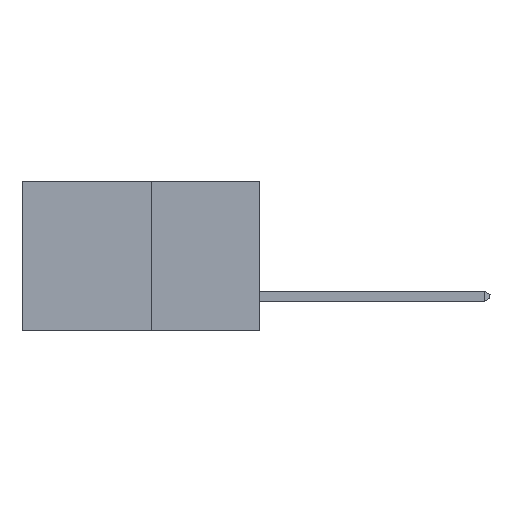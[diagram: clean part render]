
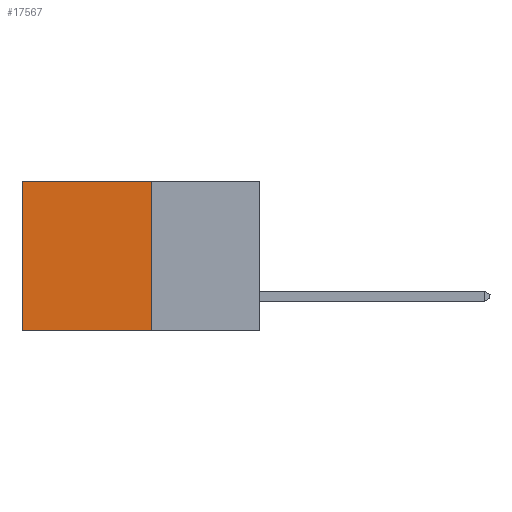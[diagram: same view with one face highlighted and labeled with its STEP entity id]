
A CAD part, left-side view. The second image highlights one B-rep face of the part: STEP entity #17567.
In plain terms, the highlighted planar face has unit normal (-1, 0, 0).
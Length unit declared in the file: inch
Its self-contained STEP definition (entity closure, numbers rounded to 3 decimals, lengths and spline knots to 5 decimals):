
#371 = CARTESIAN_POINT ( 'NONE',  ( 0.277, 0.59, 0. ) ) ;
#613 = ORIENTED_EDGE ( 'NONE', *, *, #22985, .F. ) ;
#982 = AXIS2_PLACEMENT_3D ( 'NONE', #13356, #4109, #20392 ) ;
#1443 = VECTOR ( 'NONE', #17323, 39.37008 ) ;
#1579 = VECTOR ( 'NONE', #10086, 39.37008 ) ;
#2137 = LINE ( 'NONE', #10068, #1579 ) ;
#4109 = DIRECTION ( 'NONE',  ( 1., 0., 0. ) ) ;
#4793 = CARTESIAN_POINT ( 'NONE',  ( 0.277, 0.59, -0.37 ) ) ;
#5698 = CARTESIAN_POINT ( 'NONE',  ( 0.277, 0.27, 0. ) ) ;
#8497 = EDGE_LOOP ( 'NONE', ( #13514, #21182, #613, #10067 ) ) ;
#8804 = EDGE_CURVE ( 'NONE', #21291, #21212, #9125, .T. ) ;
#9125 = LINE ( 'NONE', #29122, #25935 ) ;
#10067 = ORIENTED_EDGE ( 'NONE', *, *, #27814, .T. ) ;
#10068 = CARTESIAN_POINT ( 'NONE',  ( 0.277, 0.27, -0.37 ) ) ;
#10086 = DIRECTION ( 'NONE',  ( 0., 1., 0. ) ) ;
#10273 = EDGE_CURVE ( 'NONE', #24475, #21212, #2137, .T. ) ;
#12846 = VERTEX_POINT ( 'NONE', #28632 ) ;
#13356 = CARTESIAN_POINT ( 'NONE',  ( 0.277, 0.27, -0.37 ) ) ;
#13514 = ORIENTED_EDGE ( 'NONE', *, *, #8804, .T. ) ;
#16213 = CARTESIAN_POINT ( 'NONE',  ( 0.277, 0.27, -0.37 ) ) ;
#17323 = DIRECTION ( 'NONE',  ( 0., 1., 0. ) ) ;
#17567 = ADVANCED_FACE ( 'NONE', ( #23537 ), #17945, .F. ) ;
#17945 = PLANE ( 'NONE',  #982 ) ;
#18437 = DIRECTION ( 'NONE',  ( 0., 0., -1. ) ) ;
#18791 = LINE ( 'NONE', #16213, #24263 ) ;
#19976 = LINE ( 'NONE', #5698, #1443 ) ;
#20392 = DIRECTION ( 'NONE',  ( 0., 0., -1. ) ) ;
#21182 = ORIENTED_EDGE ( 'NONE', *, *, #10273, .F. ) ;
#21212 = VERTEX_POINT ( 'NONE', #4793 ) ;
#21291 = VERTEX_POINT ( 'NONE', #371 ) ;
#22985 = EDGE_CURVE ( 'NONE', #12846, #24475, #18791, .T. ) ;
#23537 = FACE_OUTER_BOUND ( 'NONE', #8497, .T. ) ;
#23596 = CARTESIAN_POINT ( 'NONE',  ( 0.277, 0.27, -0.37 ) ) ;
#24263 = VECTOR ( 'NONE', #18437, 39.37008 ) ;
#24475 = VERTEX_POINT ( 'NONE', #23596 ) ;
#25935 = VECTOR ( 'NONE', #29084, 39.37008 ) ;
#27814 = EDGE_CURVE ( 'NONE', #12846, #21291, #19976, .T. ) ;
#28632 = CARTESIAN_POINT ( 'NONE',  ( 0.277, 0.27, 0. ) ) ;
#29084 = DIRECTION ( 'NONE',  ( 0., 0., -1. ) ) ;
#29122 = CARTESIAN_POINT ( 'NONE',  ( 0.277, 0.59, -0.37 ) ) ;
